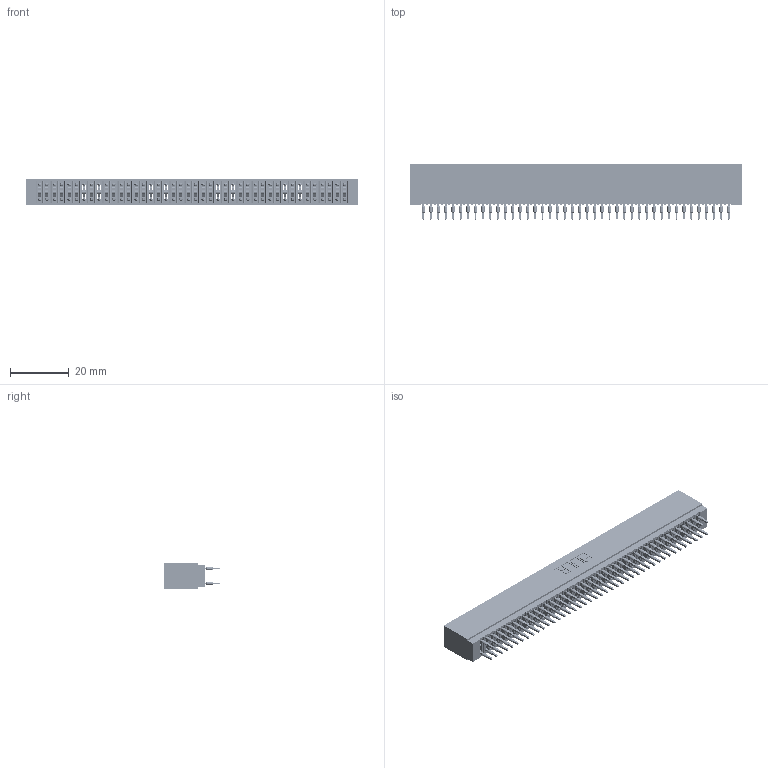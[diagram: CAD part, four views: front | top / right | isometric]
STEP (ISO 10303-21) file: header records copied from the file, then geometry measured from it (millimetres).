
FILE_DESCRIPTION (( 'STEP AP203' ), '1' );
FILE_NAME ('725-084-560-201.STEP', '2026-02-24T19:14:40', ( '' ), ( '' ), 'SwSTEP 2.0', 'SolidWorks 2023', '' );
FILE_SCHEMA (( 'CONFIG_CONTROL_DESIGN' ));
Length unit declared in the file: millimetre
Products named in the file (3): 725 Part_Insulator Option - 01; 725-084-560-201; 745-292-001_560
Assembly tree (85 placements, depth 2):
  725-084-560-201
    725 Part_Insulator Option - 01
    745-292-001_560  x84
Bounding box: 113.28 x 18.8 x 8.89 mm (x, y, z)
Volume: 9293.8 mm3; surface area: 20954.2 mm2
Topology: 85 solids, 85 shells, 8369 faces, 22892 edges, 14532 vertices
Faces by surface type: plane 4339, cylinder 1846, bspline 1680, torus 504
Entity records: 70995 total; most frequent: CARTESIAN_POINT 12817, ORIENTED_EDGE 12252, DIRECTION 10710, EDGE_CURVE 6126, LINE 5684, VECTOR 5684, VERTEX_POINT 3908, AXIS2_PLACEMENT_3D 2513
